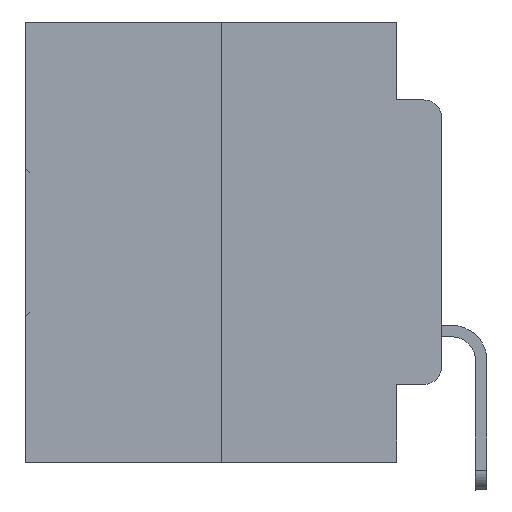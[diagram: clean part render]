
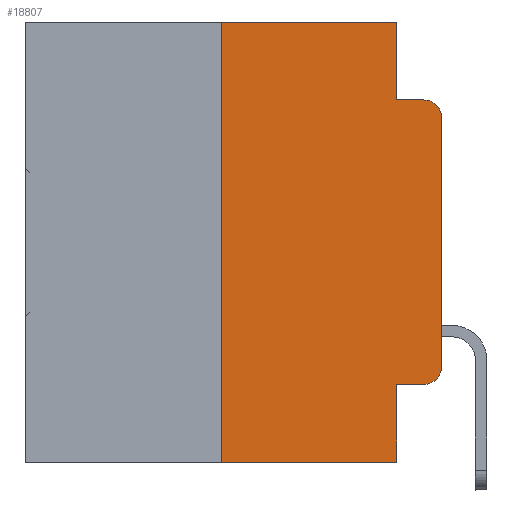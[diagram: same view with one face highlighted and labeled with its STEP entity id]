
A CAD part, left-side view. The second image highlights one B-rep face of the part: STEP entity #18807.
In plain terms, the highlighted planar face has unit normal (-1, 0, 0).
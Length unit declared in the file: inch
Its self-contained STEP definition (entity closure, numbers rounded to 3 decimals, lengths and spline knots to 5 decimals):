
#190 = DIRECTION ( 'NONE',  ( 1., 0., 0. ) ) ;
#341 = FACE_OUTER_BOUND ( 'NONE', #16998, .T. ) ;
#347 = ORIENTED_EDGE ( 'NONE', *, *, #27311, .F. ) ;
#434 = DIRECTION ( 'NONE',  ( -1., 0., 0. ) ) ;
#1072 = VECTOR ( 'NONE', #15540, 39.37008 ) ;
#1157 = CARTESIAN_POINT ( 'NONE',  ( 0., 0.051, 0. ) ) ;
#1801 = CARTESIAN_POINT ( 'NONE',  ( 0., 0.02, -0.0885 ) ) ;
#2021 = CARTESIAN_POINT ( 'NONE',  ( 0., 0., -0.3915 ) ) ;
#2318 = CARTESIAN_POINT ( 'NONE',  ( 0., 0.25, 0. ) ) ;
#2320 = DIRECTION ( 'NONE',  ( -1., 0., 0. ) ) ;
#2404 = ORIENTED_EDGE ( 'NONE', *, *, #22271, .F. ) ;
#2639 = DIRECTION ( 'NONE',  ( 0., 0., -1. ) ) ;
#2778 = LINE ( 'NONE', #7464, #8963 ) ;
#2915 = VECTOR ( 'NONE', #9813, 39.37008 ) ;
#2967 = CIRCLE ( 'NONE', #6979, 0.02 ) ;
#3740 = EDGE_CURVE ( 'NONE', #4876, #27202, #20376, .T. ) ;
#3978 = VECTOR ( 'NONE', #23080, 39.37008 ) ;
#4121 = DIRECTION ( 'NONE',  ( 0., 0., -1. ) ) ;
#4448 = VERTEX_POINT ( 'NONE', #2318 ) ;
#4591 = LINE ( 'NONE', #11184, #3978 ) ;
#4876 = VERTEX_POINT ( 'NONE', #18348 ) ;
#5247 = VERTEX_POINT ( 'NONE', #13285 ) ;
#5714 = EDGE_CURVE ( 'NONE', #23695, #24841, #8562, .T. ) ;
#5958 = CARTESIAN_POINT ( 'NONE',  ( 0., 0.051, 0. ) ) ;
#6675 = CARTESIAN_POINT ( 'NONE',  ( 0., 0.051, -0.5 ) ) ;
#6864 = VERTEX_POINT ( 'NONE', #1801 ) ;
#6979 = AXIS2_PLACEMENT_3D ( 'NONE', #16598, #2320, #2639 ) ;
#7106 = ORIENTED_EDGE ( 'NONE', *, *, #25177, .F. ) ;
#7454 = CARTESIAN_POINT ( 'NONE',  ( 0., 0.051, -0.0885 ) ) ;
#7464 = CARTESIAN_POINT ( 'NONE',  ( 0., 0., 0. ) ) ;
#7617 = DIRECTION ( 'NONE',  ( 0., 0., 1. ) ) ;
#7628 = CARTESIAN_POINT ( 'NONE',  ( 0., 0., -0.1085 ) ) ;
#8425 = EDGE_CURVE ( 'NONE', #30205, #14319, #2967, .T. ) ;
#8562 = LINE ( 'NONE', #27813, #16363 ) ;
#8963 = VECTOR ( 'NONE', #7617, 39.37008 ) ;
#9111 = ORIENTED_EDGE ( 'NONE', *, *, #20243, .T. ) ;
#9307 = DIRECTION ( 'NONE',  ( 0., 0., -1. ) ) ;
#9512 = LINE ( 'NONE', #10122, #2915 ) ;
#9813 = DIRECTION ( 'NONE',  ( 0., 0., 1. ) ) ;
#10122 = CARTESIAN_POINT ( 'NONE',  ( 0., 0.25, 0. ) ) ;
#10260 = VERTEX_POINT ( 'NONE', #7628 ) ;
#10386 = CARTESIAN_POINT ( 'NONE',  ( 0., 0.473, 0. ) ) ;
#10977 = DIRECTION ( 'NONE',  ( 0., 0., -1. ) ) ;
#11140 = ORIENTED_EDGE ( 'NONE', *, *, #3740, .F. ) ;
#11184 = CARTESIAN_POINT ( 'NONE',  ( 0., 0.051, -0.0885 ) ) ;
#11665 = ORIENTED_EDGE ( 'NONE', *, *, #12523, .F. ) ;
#12523 = EDGE_CURVE ( 'NONE', #4448, #4876, #22593, .T. ) ;
#13242 = AXIS2_PLACEMENT_3D ( 'NONE', #19467, #190, #9307 ) ;
#13285 = CARTESIAN_POINT ( 'NONE',  ( 0., 0.051, -0.4115 ) ) ;
#14301 = ORIENTED_EDGE ( 'NONE', *, *, #30075, .T. ) ;
#14319 = VERTEX_POINT ( 'NONE', #2021 ) ;
#14357 = VECTOR ( 'NONE', #24785, 39.37008 ) ;
#15131 = VECTOR ( 'NONE', #10977, 39.37008 ) ;
#15540 = DIRECTION ( 'NONE',  ( 0., -1., 0. ) ) ;
#16050 = LINE ( 'NONE', #1157, #30100 ) ;
#16363 = VECTOR ( 'NONE', #17814, 39.37008 ) ;
#16594 = CIRCLE ( 'NONE', #29588, 0.02 ) ;
#16598 = CARTESIAN_POINT ( 'NONE',  ( 0., 0.02, -0.3915 ) ) ;
#16998 = EDGE_LOOP ( 'NONE', ( #14301, #26505, #7106, #11140, #11665, #2404, #26902, #347, #9111, #21801 ) ) ;
#17814 = DIRECTION ( 'NONE',  ( 0., -1., 0. ) ) ;
#18348 = CARTESIAN_POINT ( 'NONE',  ( 0., 0.051, 0. ) ) ;
#18807 = ADVANCED_FACE ( 'NONE', ( #341 ), #26215, .F. ) ;
#19467 = CARTESIAN_POINT ( 'NONE',  ( 0., 0.473, 0. ) ) ;
#19565 = DIRECTION ( 'NONE',  ( 0., 0., -1. ) ) ;
#19971 = CARTESIAN_POINT ( 'NONE',  ( 0., 0.25, -0.5 ) ) ;
#20243 = EDGE_CURVE ( 'NONE', #5247, #30205, #29330, .T. ) ;
#20376 = LINE ( 'NONE', #5958, #15131 ) ;
#21801 = ORIENTED_EDGE ( 'NONE', *, *, #8425, .T. ) ;
#22271 = EDGE_CURVE ( 'NONE', #23695, #4448, #9512, .T. ) ;
#22593 = LINE ( 'NONE', #10386, #1072 ) ;
#22649 = CARTESIAN_POINT ( 'NONE',  ( 0., 0.02, -0.4115 ) ) ;
#23080 = DIRECTION ( 'NONE',  ( 0., -1., 0. ) ) ;
#23695 = VERTEX_POINT ( 'NONE', #19971 ) ;
#24785 = DIRECTION ( 'NONE',  ( 0., -1., 0. ) ) ;
#24841 = VERTEX_POINT ( 'NONE', #6675 ) ;
#25177 = EDGE_CURVE ( 'NONE', #27202, #6864, #4591, .T. ) ;
#26215 = PLANE ( 'NONE',  #13242 ) ;
#26505 = ORIENTED_EDGE ( 'NONE', *, *, #26800, .T. ) ;
#26800 = EDGE_CURVE ( 'NONE', #10260, #6864, #16594, .T. ) ;
#26902 = ORIENTED_EDGE ( 'NONE', *, *, #5714, .T. ) ;
#27202 = VERTEX_POINT ( 'NONE', #7454 ) ;
#27311 = EDGE_CURVE ( 'NONE', #5247, #24841, #16050, .T. ) ;
#27430 = CARTESIAN_POINT ( 'NONE',  ( 0., 0.051, -0.4115 ) ) ;
#27813 = CARTESIAN_POINT ( 'NONE',  ( 0., 0.473, -0.5 ) ) ;
#29117 = CARTESIAN_POINT ( 'NONE',  ( 0., 0.02, -0.1085 ) ) ;
#29330 = LINE ( 'NONE', #27430, #14357 ) ;
#29588 = AXIS2_PLACEMENT_3D ( 'NONE', #29117, #434, #19565 ) ;
#30075 = EDGE_CURVE ( 'NONE', #14319, #10260, #2778, .T. ) ;
#30100 = VECTOR ( 'NONE', #4121, 39.37008 ) ;
#30205 = VERTEX_POINT ( 'NONE', #22649 ) ;
